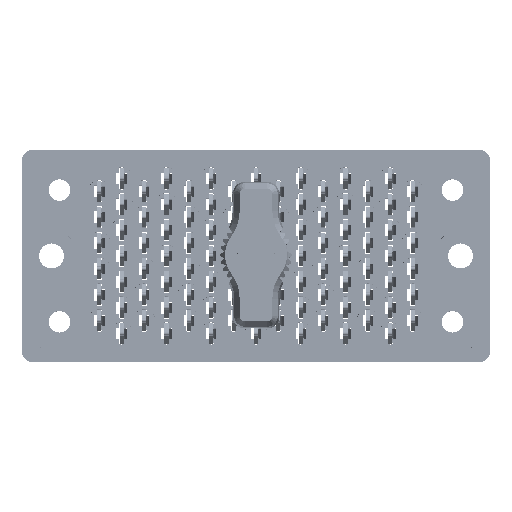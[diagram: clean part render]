
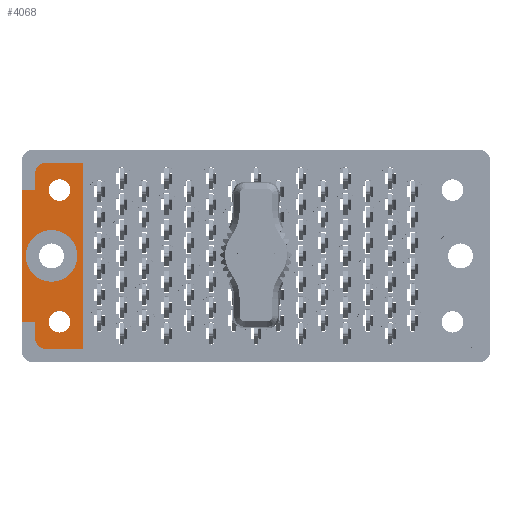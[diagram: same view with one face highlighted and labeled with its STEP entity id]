
A CAD part, top view. The second image highlights one B-rep face of the part: STEP entity #4068.
In plain terms, the highlighted planar face has unit normal (0, 0, 1).
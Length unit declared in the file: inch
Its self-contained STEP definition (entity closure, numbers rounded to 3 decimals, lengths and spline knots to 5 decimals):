
#897 = DIRECTION ( 'NONE',  ( -1., 0., 0. ) ) ;
#1238 = LINE ( 'NONE', #19066, #7535 ) ;
#1419 = CARTESIAN_POINT ( 'NONE',  ( -1.005, 0.54, -0.117 ) ) ;
#2381 = EDGE_LOOP ( 'NONE', ( #71559, #35451 ) ) ;
#3059 = ORIENTED_EDGE ( 'NONE', *, *, #25085, .T. ) ;
#3305 = VECTOR ( 'NONE', #59867, 39.37008 ) ;
#4068 = ADVANCED_FACE ( 'NONE', ( #27782, #81333, #9832, #7688 ), #16485, .T. ) ;
#4917 = DIRECTION ( 'NONE',  ( 1., 0., 0. ) ) ;
#4921 = EDGE_CURVE ( 'NONE', #33815, #11115, #1238, .T. ) ;
#5141 = CIRCLE ( 'NONE', #33019, 0.0625 ) ;
#6562 = VERTEX_POINT ( 'NONE', #49443 ) ;
#6809 = EDGE_LOOP ( 'NONE', ( #42049, #71418 ) ) ;
#6883 = VECTOR ( 'NONE', #26388, 39.37008 ) ;
#7530 = AXIS2_PLACEMENT_3D ( 'NONE', #60114, #80968, #19625 ) ;
#7535 = VECTOR ( 'NONE', #45805, 39.37008 ) ;
#7668 = DIRECTION ( 'NONE',  ( -1., 0., 0. ) ) ;
#7688 = FACE_OUTER_BOUND ( 'NONE', #47927, .T. ) ;
#7897 = AXIS2_PLACEMENT_3D ( 'NONE', #54753, #21311, #62383 ) ;
#8419 = LINE ( 'NONE', #34451, #61055 ) ;
#8538 = ORIENTED_EDGE ( 'NONE', *, *, #36854, .F. ) ;
#8611 = DIRECTION ( 'NONE',  ( 0., 0., 1. ) ) ;
#8916 = CARTESIAN_POINT ( 'NONE',  ( -1.2205, 0.478, -0.117 ) ) ;
#9245 = CARTESIAN_POINT ( 'NONE',  ( -1.005, 0.617, -0.117 ) ) ;
#9555 = EDGE_CURVE ( 'NONE', #38562, #80527, #5141, .T. ) ;
#9832 = FACE_BOUND ( 'NONE', #2381, .T. ) ;
#10832 = AXIS2_PLACEMENT_3D ( 'NONE', #15972, #57346, #69730 ) ;
#11115 = VERTEX_POINT ( 'NONE', #12572 ) ;
#11847 = DIRECTION ( 'NONE',  ( -1., 0., 0. ) ) ;
#11849 = LINE ( 'NONE', #18614, #81229 ) ;
#11943 = ORIENTED_EDGE ( 'NONE', *, *, #4921, .T. ) ;
#12558 = VERTEX_POINT ( 'NONE', #54641 ) ;
#12572 = CARTESIAN_POINT ( 'NONE',  ( -1.359, -0.3825, -0.117 ) ) ;
#12809 = CARTESIAN_POINT ( 'NONE',  ( 0., 0.3825, -0.117 ) ) ;
#12887 = CARTESIAN_POINT ( 'NONE',  ( -1.2825, 0., -0.117 ) ) ;
#13569 = CARTESIAN_POINT ( 'NONE',  ( -1.0785, 0.3825, -0.117 ) ) ;
#13848 = DIRECTION ( 'NONE',  ( 0., 0., 1. ) ) ;
#14846 = CIRCLE ( 'NONE', #7897, 0.0625 ) ;
#15032 = AXIS2_PLACEMENT_3D ( 'NONE', #32933, #53496, #52923 ) ;
#15836 = AXIS2_PLACEMENT_3D ( 'NONE', #53764, #39975, #74018 ) ;
#15972 = CARTESIAN_POINT ( 'NONE',  ( -1.1875, 0., -0.117 ) ) ;
#16270 = EDGE_CURVE ( 'NONE', #27043, #33802, #87090, .T. ) ;
#16485 = PLANE ( 'NONE',  #45609 ) ;
#18398 = AXIS2_PLACEMENT_3D ( 'NONE', #8916, #8611, #83835 ) ;
#18614 = CARTESIAN_POINT ( 'NONE',  ( 0., 0.54, -0.117 ) ) ;
#19066 = CARTESIAN_POINT ( 'NONE',  ( -1.359, 0.617, -0.117 ) ) ;
#19304 = AXIS2_PLACEMENT_3D ( 'NONE', #24716, #51413, #4917 ) ;
#19625 = DIRECTION ( 'NONE',  ( 1., 0., 0. ) ) ;
#21026 = VECTOR ( 'NONE', #42513, 39.37008 ) ;
#21311 = DIRECTION ( 'NONE',  ( 0., 0., 1. ) ) ;
#21731 = CARTESIAN_POINT ( 'NONE',  ( -1.2825, 0., -0.117 ) ) ;
#23292 = DIRECTION ( 'NONE',  ( 1., 0., 0. ) ) ;
#24716 = CARTESIAN_POINT ( 'NONE',  ( -1.141, -0.3825, -0.117 ) ) ;
#25085 = EDGE_CURVE ( 'NONE', #55415, #85738, #28402, .T. ) ;
#25527 = EDGE_LOOP ( 'NONE', ( #67297, #84283 ) ) ;
#26388 = DIRECTION ( 'NONE',  ( -1., 0., 0. ) ) ;
#27043 = VERTEX_POINT ( 'NONE', #59374 ) ;
#27782 = FACE_BOUND ( 'NONE', #6809, .T. ) ;
#28205 = VERTEX_POINT ( 'NONE', #13569 ) ;
#28224 = CARTESIAN_POINT ( 'NONE',  ( -1.0785, -0.3825, -0.117 ) ) ;
#28402 = LINE ( 'NONE', #9245, #21026 ) ;
#28511 = DIRECTION ( 'NONE',  ( 0., -1., 0. ) ) ;
#29430 = CARTESIAN_POINT ( 'NONE',  ( -1.2825, 0.3825, -0.117 ) ) ;
#30265 = CARTESIAN_POINT ( 'NONE',  ( -1.2205, 0.54, -0.117 ) ) ;
#30367 = ORIENTED_EDGE ( 'NONE', *, *, #16270, .T. ) ;
#32521 = EDGE_CURVE ( 'NONE', #6562, #11115, #8419, .T. ) ;
#32752 = EDGE_CURVE ( 'NONE', #28205, #36799, #54644, .T. ) ;
#32933 = CARTESIAN_POINT ( 'NONE',  ( -1.141, 0.3825, -0.117 ) ) ;
#33019 = AXIS2_PLACEMENT_3D ( 'NONE', #72900, #13848, #59674 ) ;
#33052 = VERTEX_POINT ( 'NONE', #30265 ) ;
#33802 = VERTEX_POINT ( 'NONE', #29430 ) ;
#33815 = VERTEX_POINT ( 'NONE', #37280 ) ;
#34451 = CARTESIAN_POINT ( 'NONE',  ( 0., -0.3825, -0.117 ) ) ;
#34871 = ORIENTED_EDGE ( 'NONE', *, *, #32521, .F. ) ;
#35128 = VERTEX_POINT ( 'NONE', #35896 ) ;
#35451 = ORIENTED_EDGE ( 'NONE', *, *, #65355, .F. ) ;
#35896 = CARTESIAN_POINT ( 'NONE',  ( -1.0375, 0., -0.117 ) ) ;
#36799 = VERTEX_POINT ( 'NONE', #67920 ) ;
#36854 = EDGE_CURVE ( 'NONE', #55415, #47674, #43564, .T. ) ;
#37280 = CARTESIAN_POINT ( 'NONE',  ( -1.359, 0.3825, -0.117 ) ) ;
#38173 = EDGE_CURVE ( 'NONE', #36799, #28205, #14846, .T. ) ;
#38562 = VERTEX_POINT ( 'NONE', #79984 ) ;
#39065 = EDGE_CURVE ( 'NONE', #80527, #38562, #78867, .T. ) ;
#39975 = DIRECTION ( 'NONE',  ( 0., 0., 1. ) ) ;
#42049 = ORIENTED_EDGE ( 'NONE', *, *, #9555, .F. ) ;
#42184 = CIRCLE ( 'NONE', #7530, 0.062 ) ;
#42513 = DIRECTION ( 'NONE',  ( 0., 1., 0. ) ) ;
#43564 = LINE ( 'NONE', #61712, #57134 ) ;
#44683 = CIRCLE ( 'NONE', #10832, 0.15 ) ;
#45609 = AXIS2_PLACEMENT_3D ( 'NONE', #69080, #76715, #23292 ) ;
#45805 = DIRECTION ( 'NONE',  ( 0., -1., 0. ) ) ;
#47674 = VERTEX_POINT ( 'NONE', #77586 ) ;
#47927 = EDGE_LOOP ( 'NONE', ( #86391, #83610, #8538, #3059, #80075, #69721, #30367, #51436, #11943, #34871 ) ) ;
#49443 = CARTESIAN_POINT ( 'NONE',  ( -1.2825, -0.3825, -0.117 ) ) ;
#49691 = EDGE_CURVE ( 'NONE', #63032, #47674, #42184, .T. ) ;
#51392 = VECTOR ( 'NONE', #28511, 39.37008 ) ;
#51413 = DIRECTION ( 'NONE',  ( 0., 0., 1. ) ) ;
#51436 = ORIENTED_EDGE ( 'NONE', *, *, #52994, .T. ) ;
#51492 = CIRCLE ( 'NONE', #15836, 0.15 ) ;
#52923 = DIRECTION ( 'NONE',  ( 1., 0., 0. ) ) ;
#52994 = EDGE_CURVE ( 'NONE', #33802, #33815, #60519, .T. ) ;
#53496 = DIRECTION ( 'NONE',  ( 0., 0., 1. ) ) ;
#53764 = CARTESIAN_POINT ( 'NONE',  ( -1.1875, 0., -0.117 ) ) ;
#54641 = CARTESIAN_POINT ( 'NONE',  ( -1.3375, 0., -0.117 ) ) ;
#54644 = CIRCLE ( 'NONE', #15032, 0.0625 ) ;
#54753 = CARTESIAN_POINT ( 'NONE',  ( -1.141, 0.3825, -0.117 ) ) ;
#55415 = VERTEX_POINT ( 'NONE', #59717 ) ;
#57134 = VECTOR ( 'NONE', #897, 39.37008 ) ;
#57346 = DIRECTION ( 'NONE',  ( 0., 0., 1. ) ) ;
#59006 = EDGE_CURVE ( 'NONE', #85738, #33052, #11849, .T. ) ;
#59374 = CARTESIAN_POINT ( 'NONE',  ( -1.2825, 0.478, -0.117 ) ) ;
#59674 = DIRECTION ( 'NONE',  ( 1., 0., 0. ) ) ;
#59717 = CARTESIAN_POINT ( 'NONE',  ( -1.005, -0.54, -0.117 ) ) ;
#59867 = DIRECTION ( 'NONE',  ( 0., -1., 0. ) ) ;
#60114 = CARTESIAN_POINT ( 'NONE',  ( -1.2205, -0.478, -0.117 ) ) ;
#60519 = LINE ( 'NONE', #12809, #6883 ) ;
#60662 = EDGE_CURVE ( 'NONE', #33052, #27043, #65151, .T. ) ;
#61055 = VECTOR ( 'NONE', #7668, 39.37008 ) ;
#61712 = CARTESIAN_POINT ( 'NONE',  ( 0., -0.54, -0.117 ) ) ;
#62119 = LINE ( 'NONE', #12887, #3305 ) ;
#62383 = DIRECTION ( 'NONE',  ( 1., 0., 0. ) ) ;
#63032 = VERTEX_POINT ( 'NONE', #86773 ) ;
#65151 = CIRCLE ( 'NONE', #18398, 0.062 ) ;
#65355 = EDGE_CURVE ( 'NONE', #12558, #35128, #44683, .T. ) ;
#67297 = ORIENTED_EDGE ( 'NONE', *, *, #38173, .F. ) ;
#67920 = CARTESIAN_POINT ( 'NONE',  ( -1.2035, 0.3825, -0.117 ) ) ;
#69080 = CARTESIAN_POINT ( 'NONE',  ( -1.359, -0.617, -0.117 ) ) ;
#69721 = ORIENTED_EDGE ( 'NONE', *, *, #60662, .T. ) ;
#69730 = DIRECTION ( 'NONE',  ( 1., 0., 0. ) ) ;
#71418 = ORIENTED_EDGE ( 'NONE', *, *, #39065, .F. ) ;
#71559 = ORIENTED_EDGE ( 'NONE', *, *, #74850, .F. ) ;
#72900 = CARTESIAN_POINT ( 'NONE',  ( -1.141, -0.3825, -0.117 ) ) ;
#74018 = DIRECTION ( 'NONE',  ( 1., 0., 0. ) ) ;
#74850 = EDGE_CURVE ( 'NONE', #35128, #12558, #51492, .T. ) ;
#76715 = DIRECTION ( 'NONE',  ( 0., 0., 1. ) ) ;
#77586 = CARTESIAN_POINT ( 'NONE',  ( -1.2205, -0.54, -0.117 ) ) ;
#78867 = CIRCLE ( 'NONE', #19304, 0.0625 ) ;
#79984 = CARTESIAN_POINT ( 'NONE',  ( -1.2035, -0.3825, -0.117 ) ) ;
#80075 = ORIENTED_EDGE ( 'NONE', *, *, #59006, .T. ) ;
#80527 = VERTEX_POINT ( 'NONE', #28224 ) ;
#80968 = DIRECTION ( 'NONE',  ( 0., 0., 1. ) ) ;
#81229 = VECTOR ( 'NONE', #11847, 39.37008 ) ;
#81333 = FACE_BOUND ( 'NONE', #25527, .T. ) ;
#83610 = ORIENTED_EDGE ( 'NONE', *, *, #49691, .T. ) ;
#83835 = DIRECTION ( 'NONE',  ( 1., 0., 0. ) ) ;
#84283 = ORIENTED_EDGE ( 'NONE', *, *, #32752, .F. ) ;
#85738 = VERTEX_POINT ( 'NONE', #1419 ) ;
#86232 = EDGE_CURVE ( 'NONE', #6562, #63032, #62119, .T. ) ;
#86391 = ORIENTED_EDGE ( 'NONE', *, *, #86232, .T. ) ;
#86773 = CARTESIAN_POINT ( 'NONE',  ( -1.2825, -0.478, -0.117 ) ) ;
#87090 = LINE ( 'NONE', #21731, #51392 ) ;
